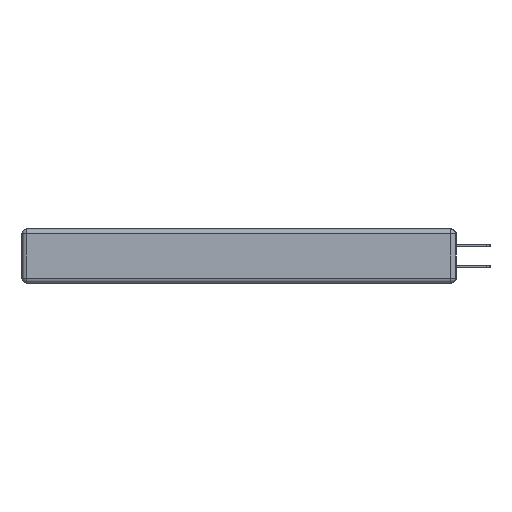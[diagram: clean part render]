
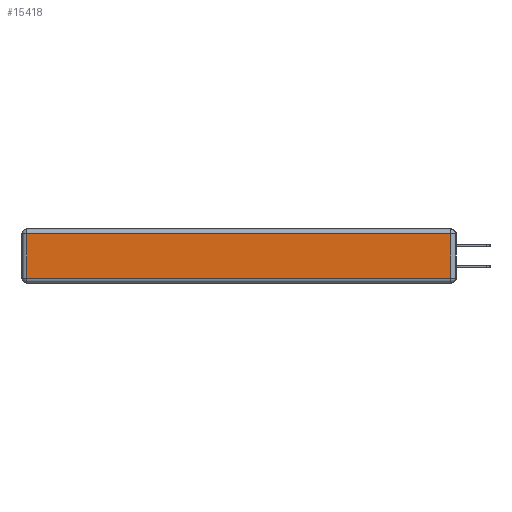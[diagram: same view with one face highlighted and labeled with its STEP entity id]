
A CAD part, left-side view. The second image highlights one B-rep face of the part: STEP entity #15418.
In plain terms, the highlighted planar face has unit normal (-1, 0, 0).
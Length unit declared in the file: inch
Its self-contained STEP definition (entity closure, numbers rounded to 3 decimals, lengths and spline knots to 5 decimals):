
#458 = VERTEX_POINT ( 'NONE', #17374 ) ;
#2746 = EDGE_CURVE ( 'NONE', #28490, #21858, #15771, .T. ) ;
#3622 = DIRECTION ( 'NONE',  ( 0., 1., 0. ) ) ;
#5279 = LINE ( 'NONE', #27631, #25820 ) ;
#5639 = CARTESIAN_POINT ( 'NONE',  ( 0., 2.72, -0.03 ) ) ;
#5746 = ORIENTED_EDGE ( 'NONE', *, *, #12345, .T. ) ;
#6176 = AXIS2_PLACEMENT_3D ( 'NONE', #21188, #18439, #20738 ) ;
#7145 = ORIENTED_EDGE ( 'NONE', *, *, #2746, .T. ) ;
#11901 = PLANE ( 'NONE',  #6176 ) ;
#12345 = EDGE_CURVE ( 'NONE', #458, #22473, #15563, .T. ) ;
#13206 = CARTESIAN_POINT ( 'NONE',  ( 0., 2.75, -0.03 ) ) ;
#13850 = DIRECTION ( 'NONE',  ( 0., -1., 0. ) ) ;
#15418 = ADVANCED_FACE ( 'NONE', ( #25492 ), #11901, .T. ) ;
#15563 = LINE ( 'NONE', #29483, #27447 ) ;
#15771 = LINE ( 'NONE', #16344, #26932 ) ;
#16344 = CARTESIAN_POINT ( 'NONE',  ( 0., 2.72, -0.343 ) ) ;
#16855 = EDGE_CURVE ( 'NONE', #22473, #28490, #26440, .T. ) ;
#17374 = CARTESIAN_POINT ( 'NONE',  ( 0., 0.03, -0.313 ) ) ;
#18193 = CARTESIAN_POINT ( 'NONE',  ( 0., 0.03, -0.03 ) ) ;
#18439 = DIRECTION ( 'NONE',  ( -1., 0., 0. ) ) ;
#20239 = DIRECTION ( 'NONE',  ( 0., 0., 1. ) ) ;
#20738 = DIRECTION ( 'NONE',  ( 0., 0., 1. ) ) ;
#21188 = CARTESIAN_POINT ( 'NONE',  ( 0., 0., -0.343 ) ) ;
#21361 = EDGE_LOOP ( 'NONE', ( #24813, #5746, #27204, #7145 ) ) ;
#21858 = VERTEX_POINT ( 'NONE', #25115 ) ;
#21905 = EDGE_CURVE ( 'NONE', #21858, #458, #5279, .T. ) ;
#22473 = VERTEX_POINT ( 'NONE', #18193 ) ;
#22623 = DIRECTION ( 'NONE',  ( 0., 0., -1. ) ) ;
#24813 = ORIENTED_EDGE ( 'NONE', *, *, #21905, .T. ) ;
#25115 = CARTESIAN_POINT ( 'NONE',  ( 0., 2.72, -0.313 ) ) ;
#25492 = FACE_OUTER_BOUND ( 'NONE', #21361, .T. ) ;
#25820 = VECTOR ( 'NONE', #13850, 39.37008 ) ;
#26102 = VECTOR ( 'NONE', #3622, 39.37008 ) ;
#26440 = LINE ( 'NONE', #13206, #26102 ) ;
#26932 = VECTOR ( 'NONE', #22623, 39.37008 ) ;
#27204 = ORIENTED_EDGE ( 'NONE', *, *, #16855, .T. ) ;
#27447 = VECTOR ( 'NONE', #20239, 39.37008 ) ;
#27631 = CARTESIAN_POINT ( 'NONE',  ( 0., 0., -0.313 ) ) ;
#28490 = VERTEX_POINT ( 'NONE', #5639 ) ;
#29483 = CARTESIAN_POINT ( 'NONE',  ( 0., 0.03, -0.343 ) ) ;
